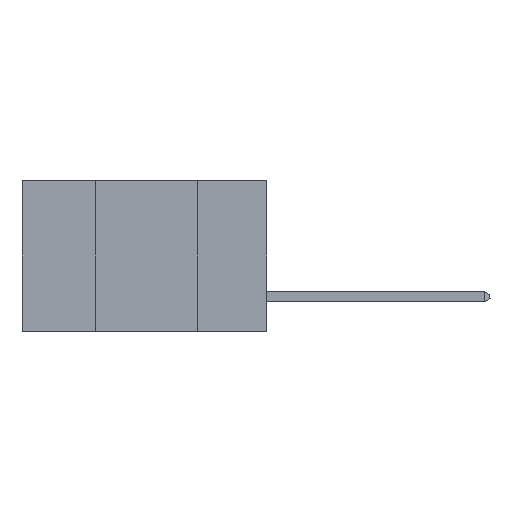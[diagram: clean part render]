
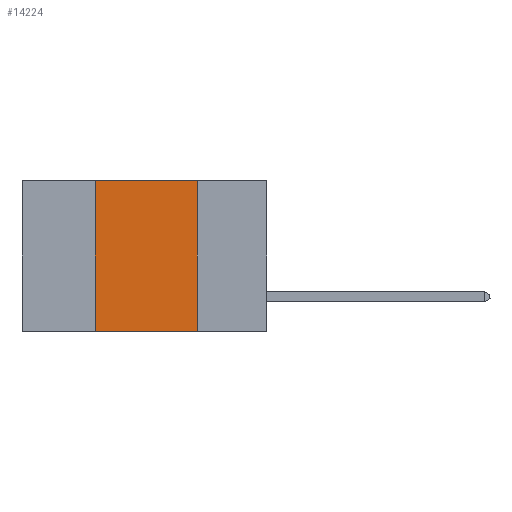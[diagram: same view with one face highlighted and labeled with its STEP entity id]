
A CAD part, left-side view. The second image highlights one B-rep face of the part: STEP entity #14224.
In plain terms, the highlighted planar face has unit normal (-1, 0, 0).
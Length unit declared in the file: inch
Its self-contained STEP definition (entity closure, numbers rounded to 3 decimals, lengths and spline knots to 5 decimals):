
#1179 = DIRECTION ( 'NONE',  ( 0., -1., 0. ) ) ;
#1465 = ORIENTED_EDGE ( 'NONE', *, *, #18902, .T. ) ;
#1815 = ORIENTED_EDGE ( 'NONE', *, *, #18189, .F. ) ;
#1817 = VECTOR ( 'NONE', #5336, 39.37008 ) ;
#1859 = CARTESIAN_POINT ( 'NONE',  ( 0., 0.6, -0.37 ) ) ;
#2086 = DIRECTION ( 'NONE',  ( 0., 0., -1. ) ) ;
#2196 = VECTOR ( 'NONE', #2987, 39.37008 ) ;
#2883 = LINE ( 'NONE', #1859, #1817 ) ;
#2987 = DIRECTION ( 'NONE',  ( 0., 0., 1. ) ) ;
#3542 = DIRECTION ( 'NONE',  ( 1., 0., 0. ) ) ;
#3789 = ORIENTED_EDGE ( 'NONE', *, *, #15911, .F. ) ;
#4709 = VERTEX_POINT ( 'NONE', #12745 ) ;
#5336 = DIRECTION ( 'NONE',  ( 0., -1., 0. ) ) ;
#7433 = EDGE_LOOP ( 'NONE', ( #1815, #3789, #8511, #1465 ) ) ;
#8511 = ORIENTED_EDGE ( 'NONE', *, *, #12778, .F. ) ;
#10255 = CARTESIAN_POINT ( 'NONE',  ( 0., 0.6, 0. ) ) ;
#10558 = FACE_OUTER_BOUND ( 'NONE', #7433, .T. ) ;
#11190 = VECTOR ( 'NONE', #1179, 39.37008 ) ;
#11769 = CARTESIAN_POINT ( 'NONE',  ( 0., 0.17, 0. ) ) ;
#12738 = CARTESIAN_POINT ( 'NONE',  ( 0., 0.17, -0.37 ) ) ;
#12745 = CARTESIAN_POINT ( 'NONE',  ( 0., 0.42, -0.37 ) ) ;
#12758 = VERTEX_POINT ( 'NONE', #12738 ) ;
#12778 = EDGE_CURVE ( 'NONE', #4709, #14088, #21673, .T. ) ;
#13456 = VECTOR ( 'NONE', #13626, 39.37008 ) ;
#13626 = DIRECTION ( 'NONE',  ( 0., 0., -1. ) ) ;
#13781 = CARTESIAN_POINT ( 'NONE',  ( 0., 0.17, 0. ) ) ;
#14088 = VERTEX_POINT ( 'NONE', #16713 ) ;
#14110 = LINE ( 'NONE', #21410, #11190 ) ;
#14224 = ADVANCED_FACE ( 'NONE', ( #10558 ), #15477, .F. ) ;
#15477 = PLANE ( 'NONE',  #20565 ) ;
#15911 = EDGE_CURVE ( 'NONE', #14088, #17008, #14110, .T. ) ;
#16713 = CARTESIAN_POINT ( 'NONE',  ( 0., 0.42, 0. ) ) ;
#17008 = VERTEX_POINT ( 'NONE', #13781 ) ;
#17917 = LINE ( 'NONE', #11769, #13456 ) ;
#18189 = EDGE_CURVE ( 'NONE', #17008, #12758, #17917, .T. ) ;
#18902 = EDGE_CURVE ( 'NONE', #4709, #12758, #2883, .T. ) ;
#20565 = AXIS2_PLACEMENT_3D ( 'NONE', #10255, #3542, #2086 ) ;
#21211 = CARTESIAN_POINT ( 'NONE',  ( 0., 0.42, 0. ) ) ;
#21410 = CARTESIAN_POINT ( 'NONE',  ( 0., 0.6, 0. ) ) ;
#21673 = LINE ( 'NONE', #21211, #2196 ) ;
